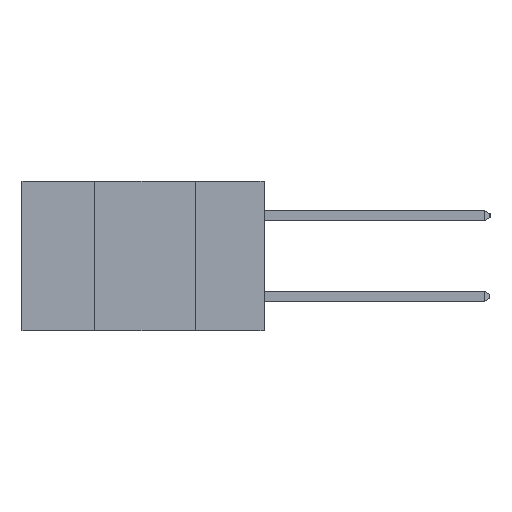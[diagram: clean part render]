
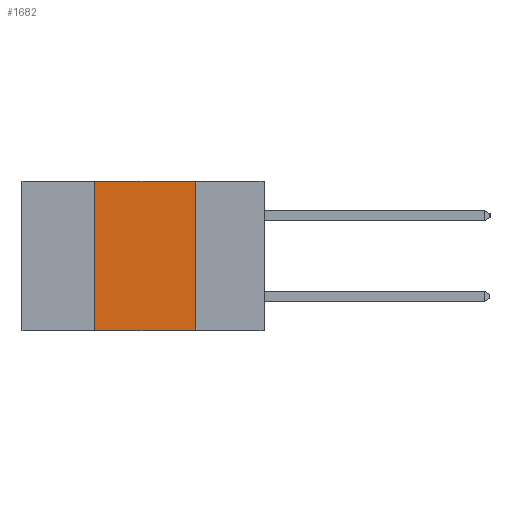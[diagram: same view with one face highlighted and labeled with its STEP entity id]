
A CAD part, left-side view. The second image highlights one B-rep face of the part: STEP entity #1682.
In plain terms, the highlighted planar face has unit normal (-1, 0, 0).
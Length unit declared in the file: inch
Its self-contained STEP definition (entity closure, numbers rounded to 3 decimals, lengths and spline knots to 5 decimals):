
#213 = DIRECTION ( 'NONE',  ( 0., 0., -1. ) ) ;
#490 = CARTESIAN_POINT ( 'NONE',  ( 0., 0.42, -0.37 ) ) ;
#812 = AXIS2_PLACEMENT_3D ( 'NONE', #8731, #7032, #5455 ) ;
#1682 = ADVANCED_FACE ( 'NONE', ( #20660 ), #20766, .F. ) ;
#2660 = EDGE_LOOP ( 'NONE', ( #3718, #18753, #17872, #21364 ) ) ;
#2953 = VERTEX_POINT ( 'NONE', #20547 ) ;
#2985 = LINE ( 'NONE', #8152, #18929 ) ;
#3149 = VERTEX_POINT ( 'NONE', #6111 ) ;
#3176 = LINE ( 'NONE', #11497, #10244 ) ;
#3678 = VERTEX_POINT ( 'NONE', #490 ) ;
#3718 = ORIENTED_EDGE ( 'NONE', *, *, #19996, .F. ) ;
#4200 = CARTESIAN_POINT ( 'NONE',  ( 0., 0.17, 0. ) ) ;
#5264 = LINE ( 'NONE', #12119, #12511 ) ;
#5455 = DIRECTION ( 'NONE',  ( 0., 0., -1. ) ) ;
#6043 = VERTEX_POINT ( 'NONE', #4200 ) ;
#6111 = CARTESIAN_POINT ( 'NONE',  ( 0., 0.42, 0. ) ) ;
#6274 = DIRECTION ( 'NONE',  ( 0., -1., 0. ) ) ;
#7032 = DIRECTION ( 'NONE',  ( 1., 0., 0. ) ) ;
#8152 = CARTESIAN_POINT ( 'NONE',  ( 0., 0.42, -0.37 ) ) ;
#8614 = VECTOR ( 'NONE', #6274, 39.37008 ) ;
#8731 = CARTESIAN_POINT ( 'NONE',  ( 0., 0.6, 0. ) ) ;
#10225 = EDGE_CURVE ( 'NONE', #3678, #3149, #2985, .T. ) ;
#10244 = VECTOR ( 'NONE', #16672, 39.37008 ) ;
#11225 = CARTESIAN_POINT ( 'NONE',  ( 0., 0.6, 0. ) ) ;
#11497 = CARTESIAN_POINT ( 'NONE',  ( 0., 0.6, -0.37 ) ) ;
#12119 = CARTESIAN_POINT ( 'NONE',  ( 0., 0.17, -0.37 ) ) ;
#12511 = VECTOR ( 'NONE', #213, 39.37008 ) ;
#14568 = LINE ( 'NONE', #11225, #8614 ) ;
#14991 = DIRECTION ( 'NONE',  ( 0., 0., 1. ) ) ;
#16672 = DIRECTION ( 'NONE',  ( 0., -1., 0. ) ) ;
#17872 = ORIENTED_EDGE ( 'NONE', *, *, #10225, .F. ) ;
#17898 = EDGE_CURVE ( 'NONE', #3678, #2953, #3176, .T. ) ;
#18753 = ORIENTED_EDGE ( 'NONE', *, *, #21366, .F. ) ;
#18929 = VECTOR ( 'NONE', #14991, 39.37008 ) ;
#19996 = EDGE_CURVE ( 'NONE', #6043, #2953, #5264, .T. ) ;
#20547 = CARTESIAN_POINT ( 'NONE',  ( 0., 0.17, -0.37 ) ) ;
#20660 = FACE_OUTER_BOUND ( 'NONE', #2660, .T. ) ;
#20766 = PLANE ( 'NONE',  #812 ) ;
#21364 = ORIENTED_EDGE ( 'NONE', *, *, #17898, .T. ) ;
#21366 = EDGE_CURVE ( 'NONE', #3149, #6043, #14568, .T. ) ;
